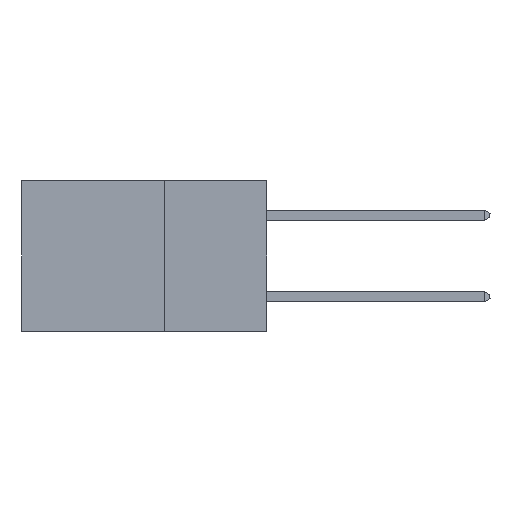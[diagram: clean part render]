
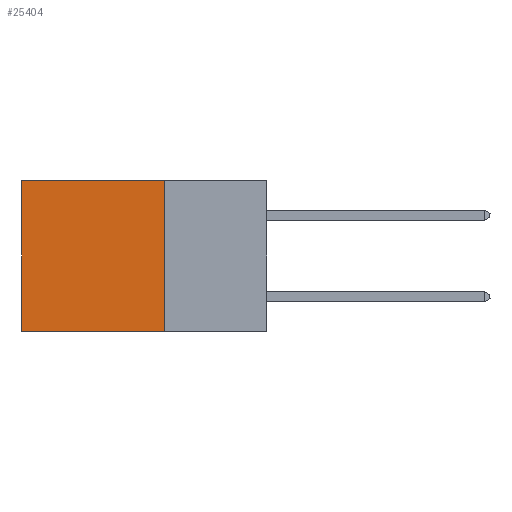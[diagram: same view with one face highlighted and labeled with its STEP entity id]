
A CAD part, left-side view. The second image highlights one B-rep face of the part: STEP entity #25404.
In plain terms, the highlighted planar face has unit normal (-1, 0, 0).
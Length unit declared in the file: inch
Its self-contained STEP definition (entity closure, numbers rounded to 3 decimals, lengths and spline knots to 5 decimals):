
#129 = LINE ( 'NONE', #1980, #14946 ) ;
#1854 = VECTOR ( 'NONE', #11990, 39.37008 ) ;
#1980 = CARTESIAN_POINT ( 'NONE',  ( 0.2875, 0.6, 0. ) ) ;
#2749 = EDGE_CURVE ( 'NONE', #17161, #14182, #37544, .T. ) ;
#2803 = CARTESIAN_POINT ( 'NONE',  ( 0.2875, 0.6, -0.37 ) ) ;
#3553 = DIRECTION ( 'NONE',  ( 0., 0., -1. ) ) ;
#5017 = DIRECTION ( 'NONE',  ( 0., 0., -1. ) ) ;
#5357 = DIRECTION ( 'NONE',  ( 0., 0., -1. ) ) ;
#7561 = VERTEX_POINT ( 'NONE', #35718 ) ;
#10419 = EDGE_CURVE ( 'NONE', #14182, #20099, #129, .T. ) ;
#11526 = CARTESIAN_POINT ( 'NONE',  ( 0.2875, 0.25, -0.37 ) ) ;
#11788 = AXIS2_PLACEMENT_3D ( 'NONE', #33409, #15309, #3553 ) ;
#11990 = DIRECTION ( 'NONE',  ( 0., 1., 0. ) ) ;
#13829 = ORIENTED_EDGE ( 'NONE', *, *, #17208, .F. ) ;
#14182 = VERTEX_POINT ( 'NONE', #23903 ) ;
#14756 = DIRECTION ( 'NONE',  ( 0., 1., 0. ) ) ;
#14946 = VECTOR ( 'NONE', #5017, 39.37008 ) ;
#15309 = DIRECTION ( 'NONE',  ( 1., 0., 0. ) ) ;
#15997 = ORIENTED_EDGE ( 'NONE', *, *, #2749, .T. ) ;
#16011 = LINE ( 'NONE', #11526, #21225 ) ;
#17161 = VERTEX_POINT ( 'NONE', #35747 ) ;
#17208 = EDGE_CURVE ( 'NONE', #7561, #20099, #16011, .T. ) ;
#20099 = VERTEX_POINT ( 'NONE', #2803 ) ;
#20581 = CARTESIAN_POINT ( 'NONE',  ( 0.2875, 0.25, 0. ) ) ;
#21225 = VECTOR ( 'NONE', #14756, 39.37008 ) ;
#22348 = ORIENTED_EDGE ( 'NONE', *, *, #23152, .F. ) ;
#23152 = EDGE_CURVE ( 'NONE', #17161, #7561, #28855, .T. ) ;
#23903 = CARTESIAN_POINT ( 'NONE',  ( 0.2875, 0.6, 0. ) ) ;
#25404 = ADVANCED_FACE ( 'NONE', ( #32039 ), #36811, .F. ) ;
#28855 = LINE ( 'NONE', #20581, #30770 ) ;
#30364 = CARTESIAN_POINT ( 'NONE',  ( 0.2875, 0.25, 0. ) ) ;
#30596 = ORIENTED_EDGE ( 'NONE', *, *, #10419, .T. ) ;
#30770 = VECTOR ( 'NONE', #5357, 39.37008 ) ;
#32039 = FACE_OUTER_BOUND ( 'NONE', #34386, .T. ) ;
#33409 = CARTESIAN_POINT ( 'NONE',  ( 0.2875, 0.25, 0. ) ) ;
#34386 = EDGE_LOOP ( 'NONE', ( #30596, #13829, #22348, #15997 ) ) ;
#35718 = CARTESIAN_POINT ( 'NONE',  ( 0.2875, 0.25, -0.37 ) ) ;
#35747 = CARTESIAN_POINT ( 'NONE',  ( 0.2875, 0.25, 0. ) ) ;
#36811 = PLANE ( 'NONE',  #11788 ) ;
#37544 = LINE ( 'NONE', #30364, #1854 ) ;
